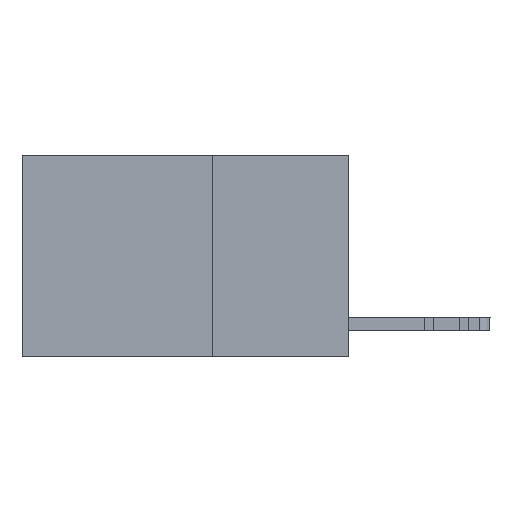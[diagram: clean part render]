
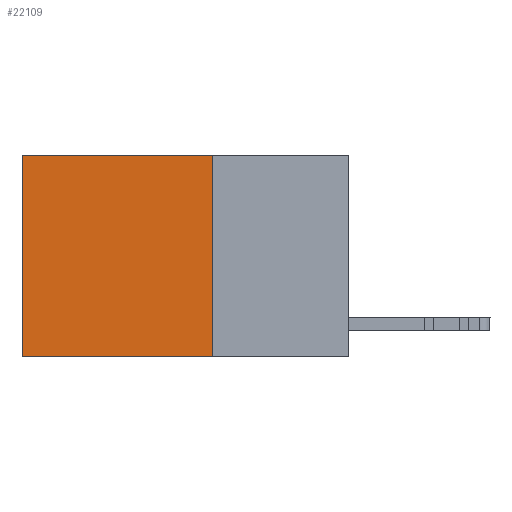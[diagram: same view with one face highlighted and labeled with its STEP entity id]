
A CAD part, left-side view. The second image highlights one B-rep face of the part: STEP entity #22109.
In plain terms, the highlighted planar face has unit normal (-1, 0, 0).
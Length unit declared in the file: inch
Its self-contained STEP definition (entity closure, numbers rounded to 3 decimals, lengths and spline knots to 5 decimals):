
#904 = LINE ( 'NONE', #5022, #12696 ) ;
#986 = ORIENTED_EDGE ( 'NONE', *, *, #13609, .F. ) ;
#1965 = ORIENTED_EDGE ( 'NONE', *, *, #3430, .F. ) ;
#2515 = LINE ( 'NONE', #14307, #14225 ) ;
#2638 = DIRECTION ( 'NONE',  ( 0., 1., 0. ) ) ;
#2939 = ORIENTED_EDGE ( 'NONE', *, *, #5561, .T. ) ;
#3430 = EDGE_CURVE ( 'NONE', #20010, #10604, #2515, .T. ) ;
#3913 = VERTEX_POINT ( 'NONE', #4387 ) ;
#4387 = CARTESIAN_POINT ( 'NONE',  ( 0.2625, 0.6, 0. ) ) ;
#4651 = PLANE ( 'NONE',  #29673 ) ;
#5022 = CARTESIAN_POINT ( 'NONE',  ( 0.2625, 0.25, 0. ) ) ;
#5561 = EDGE_CURVE ( 'NONE', #20010, #3913, #904, .T. ) ;
#6810 = VECTOR ( 'NONE', #29344, 39.37008 ) ;
#10604 = VERTEX_POINT ( 'NONE', #27938 ) ;
#11250 = LINE ( 'NONE', #21173, #22679 ) ;
#12449 = CARTESIAN_POINT ( 'NONE',  ( 0.2625, 0.25, 0. ) ) ;
#12696 = VECTOR ( 'NONE', #2638, 39.37008 ) ;
#13609 = EDGE_CURVE ( 'NONE', #10604, #29022, #11250, .T. ) ;
#14035 = DIRECTION ( 'NONE',  ( 0., 0., -1. ) ) ;
#14225 = VECTOR ( 'NONE', #27889, 39.37008 ) ;
#14307 = CARTESIAN_POINT ( 'NONE',  ( 0.2625, 0.25, 0. ) ) ;
#15775 = CARTESIAN_POINT ( 'NONE',  ( 0.2625, 0.6, 0. ) ) ;
#16428 = EDGE_LOOP ( 'NONE', ( #22998, #986, #1965, #2939 ) ) ;
#18553 = CARTESIAN_POINT ( 'NONE',  ( 0.2625, 0.25, 0. ) ) ;
#20010 = VERTEX_POINT ( 'NONE', #12449 ) ;
#21173 = CARTESIAN_POINT ( 'NONE',  ( 0.2625, 0.25, -0.37 ) ) ;
#21586 = EDGE_CURVE ( 'NONE', #3913, #29022, #25118, .T. ) ;
#22109 = ADVANCED_FACE ( 'NONE', ( #26813 ), #4651, .F. ) ;
#22679 = VECTOR ( 'NONE', #23466, 39.37008 ) ;
#22998 = ORIENTED_EDGE ( 'NONE', *, *, #21586, .T. ) ;
#23466 = DIRECTION ( 'NONE',  ( 0., 1., 0. ) ) ;
#25118 = LINE ( 'NONE', #15775, #6810 ) ;
#26660 = CARTESIAN_POINT ( 'NONE',  ( 0.2625, 0.6, -0.37 ) ) ;
#26813 = FACE_OUTER_BOUND ( 'NONE', #16428, .T. ) ;
#27625 = DIRECTION ( 'NONE',  ( 1., 0., 0. ) ) ;
#27889 = DIRECTION ( 'NONE',  ( 0., 0., -1. ) ) ;
#27938 = CARTESIAN_POINT ( 'NONE',  ( 0.2625, 0.25, -0.37 ) ) ;
#29022 = VERTEX_POINT ( 'NONE', #26660 ) ;
#29344 = DIRECTION ( 'NONE',  ( 0., 0., -1. ) ) ;
#29673 = AXIS2_PLACEMENT_3D ( 'NONE', #18553, #27625, #14035 ) ;
